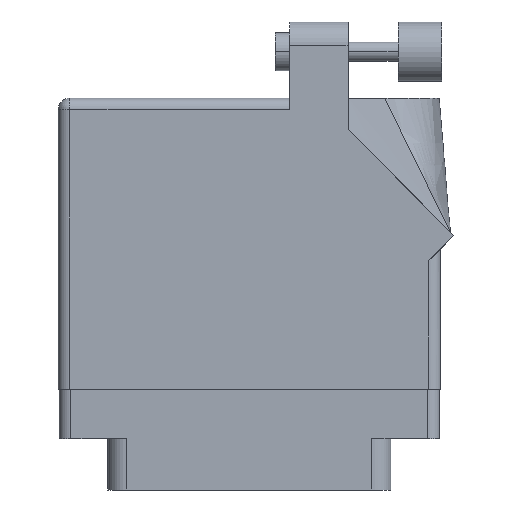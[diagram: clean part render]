
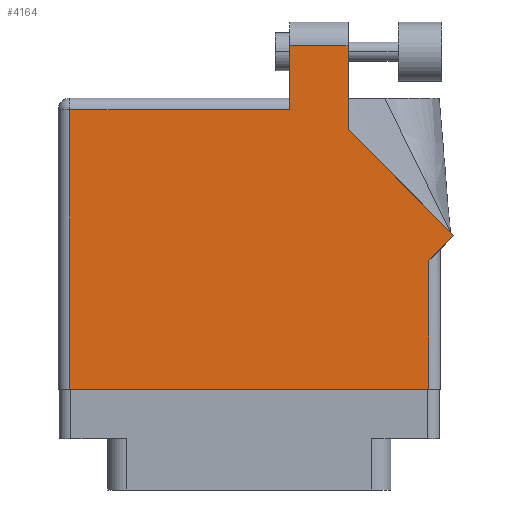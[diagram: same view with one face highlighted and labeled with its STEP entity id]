
A CAD part, front view. The second image highlights one B-rep face of the part: STEP entity #4164.
In plain terms, the highlighted face is planar.
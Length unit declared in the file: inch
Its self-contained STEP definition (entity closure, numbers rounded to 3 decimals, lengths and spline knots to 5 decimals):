
#1194 = VERTEX_POINT ( 'NONE', #14167 ) ;
#1893 = FACE_OUTER_BOUND ( 'NONE', #6906, .T. ) ;
#1968 = VECTOR ( 'NONE', #6957, 39.37008 ) ;
#3103 = CARTESIAN_POINT ( 'NONE',  ( 2.08071, 0.80771, 0. ) ) ;
#3534 = CARTESIAN_POINT ( 'NONE',  ( 2.01, 0.737, 0. ) ) ;
#3903 = AXIS2_PLACEMENT_3D ( 'NONE', #13926, #20424, #4854 ) ;
#4164 = ADVANCED_FACE ( 'NONE', ( #1893 ), #22997, .F. ) ;
#4450 = CARTESIAN_POINT ( 'NONE',  ( 1.217, 1.805, 0. ) ) ;
#4854 = DIRECTION ( 'NONE',  ( -1., 0., 0. ) ) ;
#5448 = VECTOR ( 'NONE', #26473, 39.37008 ) ;
#6891 = VERTEX_POINT ( 'NONE', #16075 ) ;
#6906 = EDGE_LOOP ( 'NONE', ( #21477, #16412, #29754, #12141, #17419, #8252, #12256, #23141, #31385 ) ) ;
#6957 = DIRECTION ( 'NONE',  ( -1., 0., 0. ) ) ;
#7028 = VERTEX_POINT ( 'NONE', #20811 ) ;
#7711 = LINE ( 'NONE', #20129, #31901 ) ;
#7881 = VERTEX_POINT ( 'NONE', #27963 ) ;
#8252 = ORIENTED_EDGE ( 'NONE', *, *, #8849, .T. ) ;
#8446 = EDGE_CURVE ( 'NONE', #20388, #15970, #14454, .T. ) ;
#8580 = EDGE_CURVE ( 'NONE', #7028, #7881, #35755, .T. ) ;
#8849 = EDGE_CURVE ( 'NONE', #11507, #20388, #7711, .T. ) ;
#9689 = DIRECTION ( 'NONE',  ( 0., -1., 0. ) ) ;
#11507 = VERTEX_POINT ( 'NONE', #13415 ) ;
#11615 = DIRECTION ( 'NONE',  ( -1., 0., 0. ) ) ;
#12141 = ORIENTED_EDGE ( 'NONE', *, *, #26096, .T. ) ;
#12256 = ORIENTED_EDGE ( 'NONE', *, *, #8446, .T. ) ;
#12587 = EDGE_CURVE ( 'NONE', #1194, #11507, #19344, .T. ) ;
#12801 = CARTESIAN_POINT ( 'NONE',  ( 1.948, 0., 0. ) ) ;
#13415 = CARTESIAN_POINT ( 'NONE',  ( 0.062, 0., 0. ) ) ;
#13670 = CARTESIAN_POINT ( 'NONE',  ( 1.948, 0.737, 0. ) ) ;
#13926 = CARTESIAN_POINT ( 'NONE',  ( 0., 1.53, 0. ) ) ;
#14167 = CARTESIAN_POINT ( 'NONE',  ( 0.062, 1.468, 0. ) ) ;
#14419 = EDGE_CURVE ( 'NONE', #20735, #25869, #37828, .T. ) ;
#14454 = LINE ( 'NONE', #13670, #33133 ) ;
#15126 = LINE ( 'NONE', #3103, #29072 ) ;
#15970 = VERTEX_POINT ( 'NONE', #37073 ) ;
#16075 = CARTESIAN_POINT ( 'NONE',  ( 2.08071, 0.80771, 0. ) ) ;
#16412 = ORIENTED_EDGE ( 'NONE', *, *, #30507, .T. ) ;
#16588 = DIRECTION ( 'NONE',  ( 1., 0., 0. ) ) ;
#17419 = ORIENTED_EDGE ( 'NONE', *, *, #12587, .T. ) ;
#19344 = LINE ( 'NONE', #31352, #22556 ) ;
#19394 = EDGE_CURVE ( 'NONE', #6891, #7028, #15126, .T. ) ;
#20129 = CARTESIAN_POINT ( 'NONE',  ( 0., 0., 0. ) ) ;
#20285 = EDGE_CURVE ( 'NONE', #15970, #6891, #21673, .T. ) ;
#20388 = VERTEX_POINT ( 'NONE', #12801 ) ;
#20424 = DIRECTION ( 'NONE',  ( 0., 0., -1. ) ) ;
#20735 = VERTEX_POINT ( 'NONE', #4450 ) ;
#20811 = CARTESIAN_POINT ( 'NONE',  ( 1.524, 1.36442, 0. ) ) ;
#21477 = ORIENTED_EDGE ( 'NONE', *, *, #8580, .T. ) ;
#21673 = LINE ( 'NONE', #3534, #28420 ) ;
#21949 = CARTESIAN_POINT ( 'NONE',  ( 1.217, 1.805, 0. ) ) ;
#22556 = VECTOR ( 'NONE', #9689, 39.37008 ) ;
#22997 = PLANE ( 'NONE',  #3903 ) ;
#23141 = ORIENTED_EDGE ( 'NONE', *, *, #20285, .T. ) ;
#25869 = VERTEX_POINT ( 'NONE', #36503 ) ;
#26096 = EDGE_CURVE ( 'NONE', #25869, #1194, #32914, .T. ) ;
#26473 = DIRECTION ( 'NONE',  ( 0., 1., 0. ) ) ;
#26801 = CARTESIAN_POINT ( 'NONE',  ( 0., 1.468, 0. ) ) ;
#27150 = DIRECTION ( 'NONE',  ( -0.707, 0.707, 0. ) ) ;
#27963 = CARTESIAN_POINT ( 'NONE',  ( 1.524, 1.805, 0. ) ) ;
#28172 = VECTOR ( 'NONE', #11615, 39.37008 ) ;
#28420 = VECTOR ( 'NONE', #30735, 39.37008 ) ;
#28938 = CARTESIAN_POINT ( 'NONE',  ( 1.217, 1.53, 0. ) ) ;
#29072 = VECTOR ( 'NONE', #27150, 39.37008 ) ;
#29222 = DIRECTION ( 'NONE',  ( 0., 1., 0. ) ) ;
#29754 = ORIENTED_EDGE ( 'NONE', *, *, #14419, .T. ) ;
#30022 = CARTESIAN_POINT ( 'NONE',  ( 1.524, 1.36442, 0. ) ) ;
#30507 = EDGE_CURVE ( 'NONE', #7881, #20735, #33594, .T. ) ;
#30735 = DIRECTION ( 'NONE',  ( 0.707, 0.707, 0. ) ) ;
#30847 = VECTOR ( 'NONE', #31896, 39.37008 ) ;
#31352 = CARTESIAN_POINT ( 'NONE',  ( 0.062, 0., 0. ) ) ;
#31385 = ORIENTED_EDGE ( 'NONE', *, *, #19394, .T. ) ;
#31896 = DIRECTION ( 'NONE',  ( 0., -1., 0. ) ) ;
#31901 = VECTOR ( 'NONE', #16588, 39.37008 ) ;
#32914 = LINE ( 'NONE', #26801, #28172 ) ;
#33133 = VECTOR ( 'NONE', #29222, 39.37008 ) ;
#33594 = LINE ( 'NONE', #21949, #1968 ) ;
#35755 = LINE ( 'NONE', #30022, #5448 ) ;
#36503 = CARTESIAN_POINT ( 'NONE',  ( 1.217, 1.468, 0. ) ) ;
#37073 = CARTESIAN_POINT ( 'NONE',  ( 1.948, 0.675, 0. ) ) ;
#37828 = LINE ( 'NONE', #28938, #30847 ) ;
